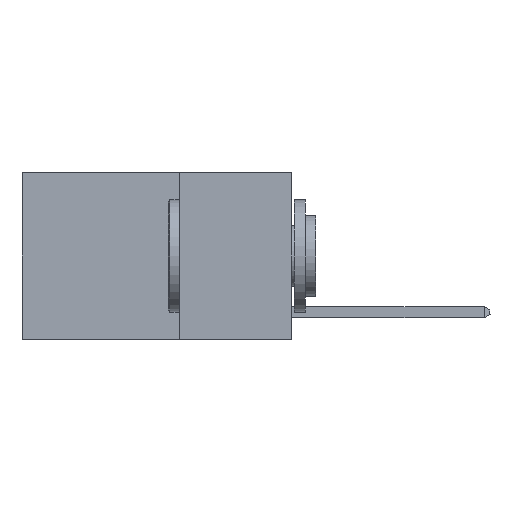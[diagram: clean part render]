
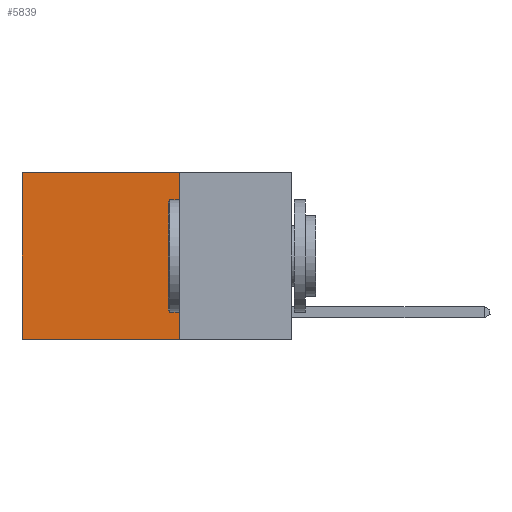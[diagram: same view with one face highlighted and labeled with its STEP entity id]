
A CAD part, left-side view. The second image highlights one B-rep face of the part: STEP entity #5839.
In plain terms, the highlighted planar face has unit normal (-1, 0, 0).
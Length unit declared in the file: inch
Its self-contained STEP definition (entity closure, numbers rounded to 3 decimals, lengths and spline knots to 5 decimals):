
#970 = DIRECTION ( 'NONE',  ( 0., 0., -1. ) ) ;
#1363 = VECTOR ( 'NONE', #24760, 39.37008 ) ;
#1457 = LINE ( 'NONE', #28315, #19946 ) ;
#2138 = CARTESIAN_POINT ( 'NONE',  ( 0.2625, 0.25, 0. ) ) ;
#2530 = VERTEX_POINT ( 'NONE', #11355 ) ;
#3212 = EDGE_CURVE ( 'NONE', #18777, #2530, #8147, .T. ) ;
#3392 = CARTESIAN_POINT ( 'NONE',  ( 0.2625, 0.25, -0.37 ) ) ;
#3989 = EDGE_LOOP ( 'NONE', ( #11258, #22215, #27929, #21866 ) ) ;
#4949 = CARTESIAN_POINT ( 'NONE',  ( 0.2625, 0.25, 0. ) ) ;
#5839 = ADVANCED_FACE ( 'NONE', ( #24815 ), #21418, .F. ) ;
#6010 = EDGE_CURVE ( 'NONE', #2530, #14320, #14281, .T. ) ;
#8147 = LINE ( 'NONE', #4949, #1363 ) ;
#8262 = CARTESIAN_POINT ( 'NONE',  ( 0.2625, 0.25, 0. ) ) ;
#9141 = DIRECTION ( 'NONE',  ( 0., 0., -1. ) ) ;
#10508 = DIRECTION ( 'NONE',  ( 1., 0., 0. ) ) ;
#11258 = ORIENTED_EDGE ( 'NONE', *, *, #6010, .T. ) ;
#11355 = CARTESIAN_POINT ( 'NONE',  ( 0.2625, 0.6, 0. ) ) ;
#12176 = VERTEX_POINT ( 'NONE', #3392 ) ;
#12413 = EDGE_CURVE ( 'NONE', #12176, #14320, #1457, .T. ) ;
#14281 = LINE ( 'NONE', #24421, #25809 ) ;
#14320 = VERTEX_POINT ( 'NONE', #15009 ) ;
#15009 = CARTESIAN_POINT ( 'NONE',  ( 0.2625, 0.6, -0.37 ) ) ;
#15102 = LINE ( 'NONE', #27455, #15783 ) ;
#15783 = VECTOR ( 'NONE', #970, 39.37008 ) ;
#17543 = DIRECTION ( 'NONE',  ( 0., 1., 0. ) ) ;
#18777 = VERTEX_POINT ( 'NONE', #2138 ) ;
#19946 = VECTOR ( 'NONE', #17543, 39.37008 ) ;
#21418 = PLANE ( 'NONE',  #23337 ) ;
#21791 = EDGE_CURVE ( 'NONE', #18777, #12176, #15102, .T. ) ;
#21866 = ORIENTED_EDGE ( 'NONE', *, *, #3212, .T. ) ;
#22215 = ORIENTED_EDGE ( 'NONE', *, *, #12413, .F. ) ;
#23337 = AXIS2_PLACEMENT_3D ( 'NONE', #8262, #10508, #25735 ) ;
#24421 = CARTESIAN_POINT ( 'NONE',  ( 0.2625, 0.6, 0. ) ) ;
#24760 = DIRECTION ( 'NONE',  ( 0., 1., 0. ) ) ;
#24815 = FACE_OUTER_BOUND ( 'NONE', #3989, .T. ) ;
#25735 = DIRECTION ( 'NONE',  ( 0., 0., -1. ) ) ;
#25809 = VECTOR ( 'NONE', #9141, 39.37008 ) ;
#27455 = CARTESIAN_POINT ( 'NONE',  ( 0.2625, 0.25, 0. ) ) ;
#27929 = ORIENTED_EDGE ( 'NONE', *, *, #21791, .F. ) ;
#28315 = CARTESIAN_POINT ( 'NONE',  ( 0.2625, 0.25, -0.37 ) ) ;
